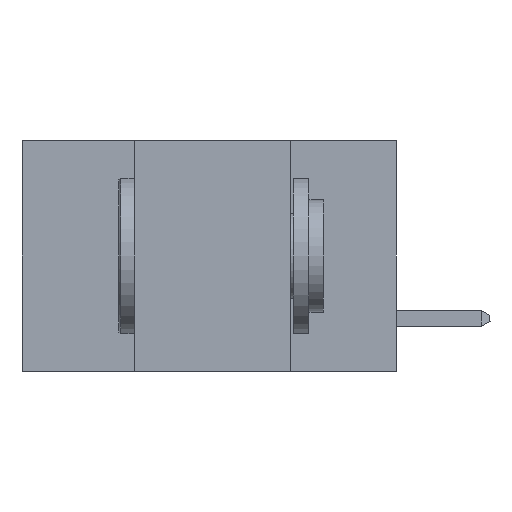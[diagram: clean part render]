
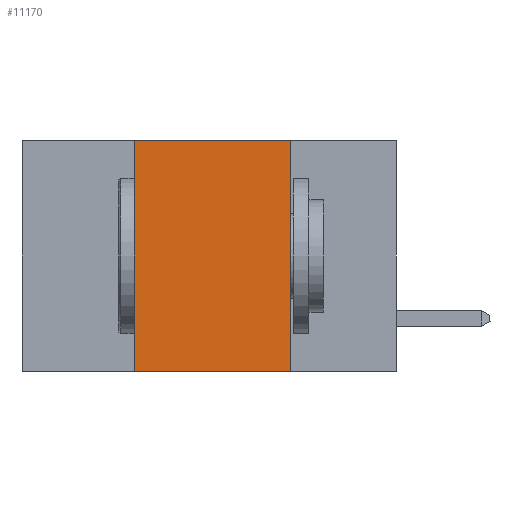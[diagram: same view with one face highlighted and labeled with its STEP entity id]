
A CAD part, left-side view. The second image highlights one B-rep face of the part: STEP entity #11170.
In plain terms, the highlighted planar face has unit normal (-1, 0, 0).
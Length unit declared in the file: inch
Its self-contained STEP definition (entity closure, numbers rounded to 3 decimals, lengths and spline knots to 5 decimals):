
#153 = VERTEX_POINT ( 'NONE', #10308 ) ;
#252 = CARTESIAN_POINT ( 'NONE',  ( 0., 0.42, 0. ) ) ;
#268 = DIRECTION ( 'NONE',  ( 0., 0., -1. ) ) ;
#660 = VECTOR ( 'NONE', #12389, 39.37008 ) ;
#1273 = DIRECTION ( 'NONE',  ( 0., 0., 1. ) ) ;
#1335 = ORIENTED_EDGE ( 'NONE', *, *, #5613, .F. ) ;
#1390 = ORIENTED_EDGE ( 'NONE', *, *, #9389, .F. ) ;
#1397 = VERTEX_POINT ( 'NONE', #2003 ) ;
#1440 = ORIENTED_EDGE ( 'NONE', *, *, #9901, .F. ) ;
#1452 = LINE ( 'NONE', #252, #4609 ) ;
#1702 = ORIENTED_EDGE ( 'NONE', *, *, #12514, .T. ) ;
#1820 = VERTEX_POINT ( 'NONE', #12866 ) ;
#2003 = CARTESIAN_POINT ( 'NONE',  ( 0., 0.17, -0.37 ) ) ;
#3210 = LINE ( 'NONE', #11704, #8257 ) ;
#4609 = VECTOR ( 'NONE', #1273, 39.37008 ) ;
#5271 = VECTOR ( 'NONE', #7656, 39.37008 ) ;
#5613 = EDGE_CURVE ( 'NONE', #153, #1397, #11694, .T. ) ;
#5902 = AXIS2_PLACEMENT_3D ( 'NONE', #10426, #6533, #268 ) ;
#6000 = VERTEX_POINT ( 'NONE', #7056 ) ;
#6521 = LINE ( 'NONE', #9600, #5271 ) ;
#6533 = DIRECTION ( 'NONE',  ( 1., 0., 0. ) ) ;
#6867 = DIRECTION ( 'NONE',  ( 0., -1., 0. ) ) ;
#7056 = CARTESIAN_POINT ( 'NONE',  ( 0., 0.42, 0. ) ) ;
#7656 = DIRECTION ( 'NONE',  ( 0., -1., 0. ) ) ;
#8257 = VECTOR ( 'NONE', #6867, 39.37008 ) ;
#8701 = EDGE_LOOP ( 'NONE', ( #1335, #1390, #1440, #1702 ) ) ;
#9224 = FACE_OUTER_BOUND ( 'NONE', #8701, .T. ) ;
#9389 = EDGE_CURVE ( 'NONE', #6000, #153, #6521, .T. ) ;
#9600 = CARTESIAN_POINT ( 'NONE',  ( 0., 0.6, 0. ) ) ;
#9901 = EDGE_CURVE ( 'NONE', #1820, #6000, #1452, .T. ) ;
#10308 = CARTESIAN_POINT ( 'NONE',  ( 0., 0.17, 0. ) ) ;
#10426 = CARTESIAN_POINT ( 'NONE',  ( 0., 0.6, 0. ) ) ;
#11170 = ADVANCED_FACE ( 'NONE', ( #9224 ), #12319, .F. ) ;
#11455 = CARTESIAN_POINT ( 'NONE',  ( 0., 0.17, 0. ) ) ;
#11694 = LINE ( 'NONE', #11455, #660 ) ;
#11704 = CARTESIAN_POINT ( 'NONE',  ( 0., 0.6, -0.37 ) ) ;
#12319 = PLANE ( 'NONE',  #5902 ) ;
#12389 = DIRECTION ( 'NONE',  ( 0., 0., -1. ) ) ;
#12514 = EDGE_CURVE ( 'NONE', #1820, #1397, #3210, .T. ) ;
#12866 = CARTESIAN_POINT ( 'NONE',  ( 0., 0.42, -0.37 ) ) ;
